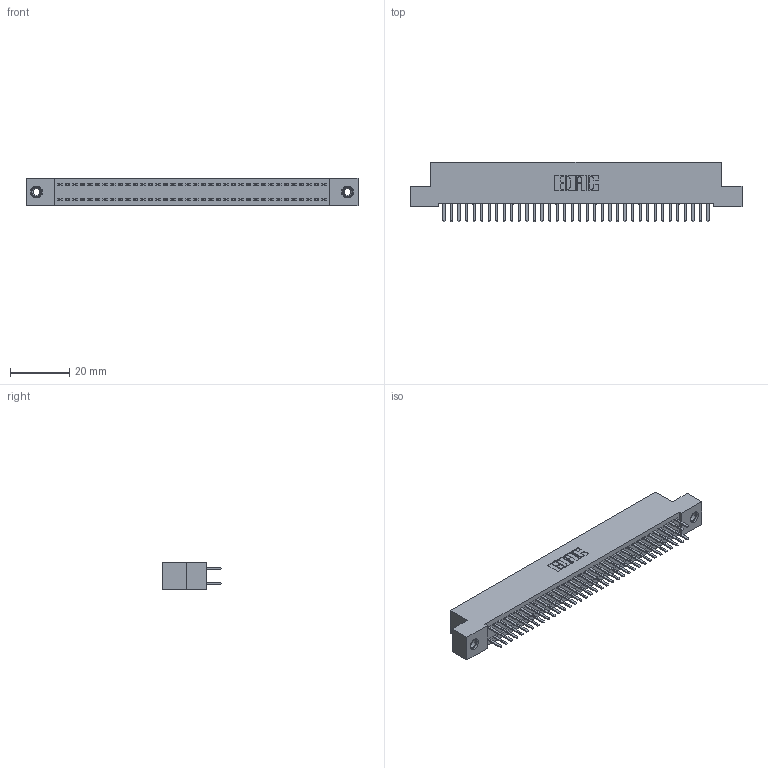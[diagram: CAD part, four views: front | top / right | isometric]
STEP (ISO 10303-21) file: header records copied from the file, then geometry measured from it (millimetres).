
FILE_DESCRIPTION (( 'STEP AP203' ), '1' );
FILE_NAME ('342-072-520-208.STEP', '2019-10-03T16:27:12', ( '' ), ( '' ), 'SwSTEP 2.0', 'SolidWorks 2016', '' );
FILE_SCHEMA (( 'CONFIG_CONTROL_DESIGN' ));
Length unit declared in the file: inch
Products named in the file (4): 345-292-001_345-293-120; 345-250-001_345-250-003-102; 342-072-520-208; 342 Part_TI
Assembly tree (75 placements, depth 2):
  342-072-520-208
    342 Part_TI
    345-292-001_345-293-120  x72
    345-250-001_345-250-003-102  x2
Bounding box: 111.76 x 20.02 x 9.4 mm (x, y, z)
Volume: 9975.9 mm3; surface area: 16026 mm2
Topology: 75 solids, 75 shells, 4202 faces, 12171 edges, 7914 vertices
Faces by surface type: plane 2834, cylinder 1352, cone 12, torus 4
Entity records: 25104 total; most frequent: CARTESIAN_POINT 4161, ORIENTED_EDGE 4078, DIRECTION 3585, EDGE_CURVE 2039, LINE 1887, VECTOR 1887, VERTEX_POINT 1352, AXIS2_PLACEMENT_3D 849
